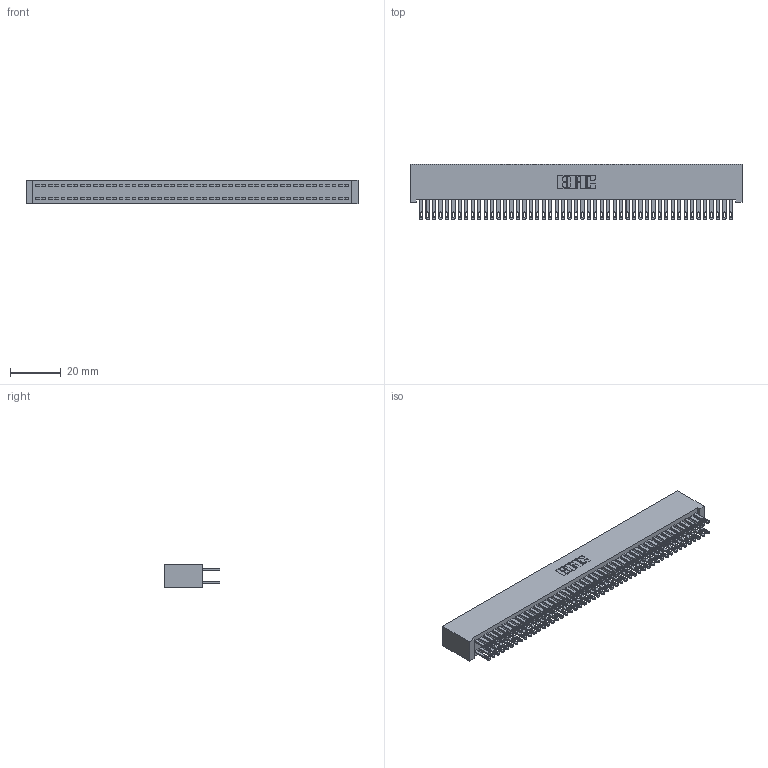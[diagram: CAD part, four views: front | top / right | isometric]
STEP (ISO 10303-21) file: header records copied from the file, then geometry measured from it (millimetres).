
FILE_DESCRIPTION (( 'STEP AP203' ), '1' );
FILE_NAME ('342-098-500-201.STEP', '2018-08-14T03:34:04', ( '' ), ( '' ), 'SwSTEP 2.0', 'SolidWorks 2016', '' );
FILE_SCHEMA (( 'CONFIG_CONTROL_DESIGN' ));
Length unit declared in the file: inch
Products named in the file (3): 342 Part_Lugless; 345-292-001_345-293-100; 342-098-500-201
Assembly tree (99 placements, depth 2):
  342-098-500-201
    342 Part_Lugless
    345-292-001_345-293-100  x98
Bounding box: 130.71 x 21.85 x 9.4 mm (x, y, z)
Volume: 12516.2 mm3; surface area: 21930.3 mm2
Topology: 99 solids, 99 shells, 4806 faces, 14681 edges, 9786 vertices
Faces by surface type: plane 3002, cylinder 1804
Entity records: 30139 total; most frequent: CARTESIAN_POINT 4982, ORIENTED_EDGE 4918, DIRECTION 4239, EDGE_CURVE 2459, LINE 2335, VECTOR 2335, VERTEX_POINT 1638, AXIS2_PLACEMENT_3D 952
